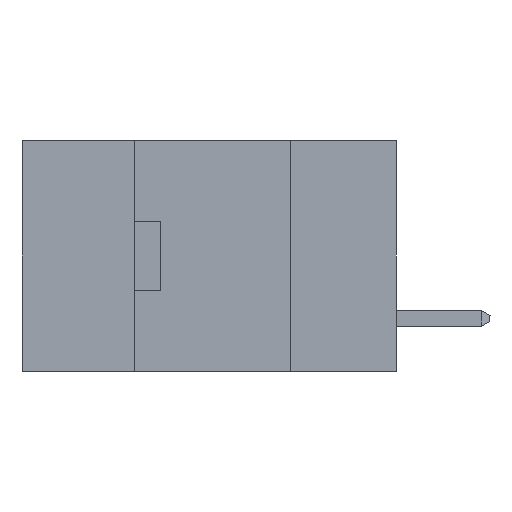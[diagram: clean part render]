
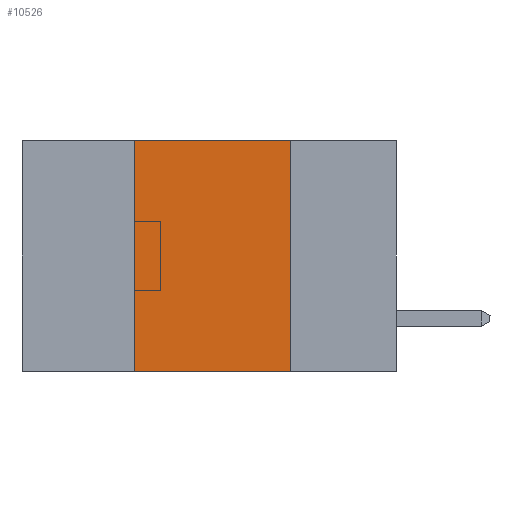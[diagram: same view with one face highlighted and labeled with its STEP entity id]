
A CAD part, left-side view. The second image highlights one B-rep face of the part: STEP entity #10526.
In plain terms, the highlighted planar face has unit normal (-1, 0, 0).
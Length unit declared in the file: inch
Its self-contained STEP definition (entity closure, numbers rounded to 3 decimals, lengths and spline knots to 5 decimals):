
#555 = CARTESIAN_POINT ( 'NONE',  ( 0., 0.42, -0.37 ) ) ;
#1444 = PLANE ( 'NONE',  #8086 ) ;
#2535 = ORIENTED_EDGE ( 'NONE', *, *, #10471, .F. ) ;
#2845 = CARTESIAN_POINT ( 'NONE',  ( 0., 0.17, 0. ) ) ;
#2913 = CARTESIAN_POINT ( 'NONE',  ( 0., 0.6, -0.37 ) ) ;
#2943 = DIRECTION ( 'NONE',  ( 0., -1., 0. ) ) ;
#3374 = EDGE_CURVE ( 'NONE', #18111, #26054, #22150, .T. ) ;
#4962 = EDGE_CURVE ( 'NONE', #14422, #22363, #21618, .T. ) ;
#5252 = EDGE_CURVE ( 'NONE', #14422, #26054, #9362, .T. ) ;
#5601 = VECTOR ( 'NONE', #6737, 39.37008 ) ;
#5937 = VECTOR ( 'NONE', #2943, 39.37008 ) ;
#6737 = DIRECTION ( 'NONE',  ( 0., 0., 1. ) ) ;
#8086 = AXIS2_PLACEMENT_3D ( 'NONE', #25899, #9662, #9137 ) ;
#9137 = DIRECTION ( 'NONE',  ( 0., 0., -1. ) ) ;
#9362 = LINE ( 'NONE', #2913, #23381 ) ;
#9469 = CARTESIAN_POINT ( 'NONE',  ( 0., 0.42, 0. ) ) ;
#9662 = DIRECTION ( 'NONE',  ( 1., 0., 0. ) ) ;
#9797 = CARTESIAN_POINT ( 'NONE',  ( 0., 0.17, -0.37 ) ) ;
#10471 = EDGE_CURVE ( 'NONE', #22363, #18111, #15017, .T. ) ;
#10526 = ADVANCED_FACE ( 'NONE', ( #11131 ), #1444, .F. ) ;
#11131 = FACE_OUTER_BOUND ( 'NONE', #16535, .T. ) ;
#13099 = ORIENTED_EDGE ( 'NONE', *, *, #5252, .T. ) ;
#14422 = VERTEX_POINT ( 'NONE', #555 ) ;
#15017 = LINE ( 'NONE', #17177, #5937 ) ;
#15934 = ORIENTED_EDGE ( 'NONE', *, *, #3374, .F. ) ;
#16535 = EDGE_LOOP ( 'NONE', ( #15934, #2535, #16571, #13099 ) ) ;
#16571 = ORIENTED_EDGE ( 'NONE', *, *, #4962, .F. ) ;
#17177 = CARTESIAN_POINT ( 'NONE',  ( 0., 0.6, 0. ) ) ;
#17284 = DIRECTION ( 'NONE',  ( 0., -1., 0. ) ) ;
#17984 = DIRECTION ( 'NONE',  ( 0., 0., -1. ) ) ;
#18111 = VERTEX_POINT ( 'NONE', #2845 ) ;
#21618 = LINE ( 'NONE', #25134, #5601 ) ;
#22150 = LINE ( 'NONE', #9797, #26075 ) ;
#22363 = VERTEX_POINT ( 'NONE', #9469 ) ;
#23381 = VECTOR ( 'NONE', #17284, 39.37008 ) ;
#23510 = CARTESIAN_POINT ( 'NONE',  ( 0., 0.17, -0.37 ) ) ;
#25134 = CARTESIAN_POINT ( 'NONE',  ( 0., 0.42, -0.37 ) ) ;
#25899 = CARTESIAN_POINT ( 'NONE',  ( 0., 0.6, 0. ) ) ;
#26054 = VERTEX_POINT ( 'NONE', #23510 ) ;
#26075 = VECTOR ( 'NONE', #17984, 39.37008 ) ;
